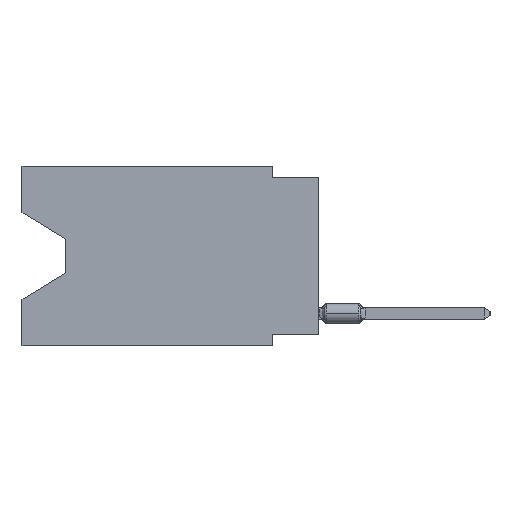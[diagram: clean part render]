
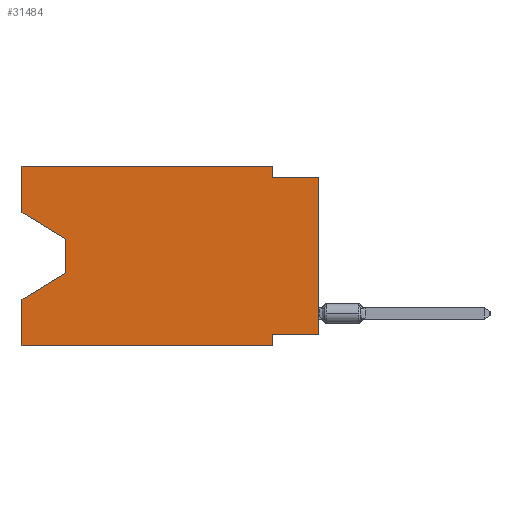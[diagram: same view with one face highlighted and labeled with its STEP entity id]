
A CAD part, left-side view. The second image highlights one B-rep face of the part: STEP entity #31484.
In plain terms, the highlighted planar face has unit normal (-1, 0, 0).
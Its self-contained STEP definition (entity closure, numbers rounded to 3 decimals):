
#155 = ORIENTED_EDGE ( 'NONE', *, *, #20727, .F. ) ;
#214 = AXIS2_PLACEMENT_3D ( 'NONE', #3123, #30117, #22687 ) ;
#402 = ORIENTED_EDGE ( 'NONE', *, *, #4136, .T. ) ;
#1003 = ORIENTED_EDGE ( 'NONE', *, *, #9504, .F. ) ;
#1324 = VECTOR ( 'NONE', #27673, 1000. ) ;
#1703 = LINE ( 'NONE', #6898, #7057 ) ;
#1825 = LINE ( 'NONE', #4101, #21482 ) ;
#2142 = DIRECTION ( 'NONE',  ( 0., 0., 1. ) ) ;
#2605 = CARTESIAN_POINT ( 'NONE',  ( 0., 16.383, 0. ) ) ;
#3123 = CARTESIAN_POINT ( 'NONE',  ( 0., 16.383, 0. ) ) ;
#3642 = VERTEX_POINT ( 'NONE', #16139 ) ;
#3894 = VECTOR ( 'NONE', #19125, 1000. ) ;
#3971 = DIRECTION ( 'NONE',  ( 0., -0.855, -0.519 ) ) ;
#4101 = CARTESIAN_POINT ( 'NONE',  ( 0., 16.383, 0. ) ) ;
#4132 = DIRECTION ( 'NONE',  ( 0., 0.855, -0.519 ) ) ;
#4136 = EDGE_CURVE ( 'NONE', #3642, #24219, #1703, .T. ) ;
#4231 = VERTEX_POINT ( 'NONE', #31960 ) ;
#4396 = LINE ( 'NONE', #24422, #4409 ) ;
#4409 = VECTOR ( 'NONE', #12322, 1000. ) ;
#5111 = EDGE_CURVE ( 'NONE', #23301, #28499, #31441, .T. ) ;
#5326 = VECTOR ( 'NONE', #3971, 1000. ) ;
#5373 = EDGE_CURVE ( 'NONE', #23481, #8202, #28333, .T. ) ;
#6181 = LINE ( 'NONE', #30898, #21129 ) ;
#6248 = CARTESIAN_POINT ( 'NONE',  ( 0., 2.54, -0.635 ) ) ;
#6339 = CARTESIAN_POINT ( 'NONE',  ( 0., 2.54, -9.271 ) ) ;
#6762 = CARTESIAN_POINT ( 'NONE',  ( 0., 0., -9.271 ) ) ;
#6898 = CARTESIAN_POINT ( 'NONE',  ( 0., 0., 0. ) ) ;
#7057 = VECTOR ( 'NONE', #25969, 1000. ) ;
#8122 = VERTEX_POINT ( 'NONE', #19099 ) ;
#8202 = VERTEX_POINT ( 'NONE', #22003 ) ;
#8298 = CARTESIAN_POINT ( 'NONE',  ( 0., 16.383, -7.36 ) ) ;
#8911 = VERTEX_POINT ( 'NONE', #6248 ) ;
#8922 = DIRECTION ( 'NONE',  ( 0., 0., -1. ) ) ;
#9165 = VERTEX_POINT ( 'NONE', #8298 ) ;
#9504 = EDGE_CURVE ( 'NONE', #13565, #8122, #4396, .T. ) ;
#11498 = ORIENTED_EDGE ( 'NONE', *, *, #24929, .F. ) ;
#12017 = ORIENTED_EDGE ( 'NONE', *, *, #30044, .T. ) ;
#12322 = DIRECTION ( 'NONE',  ( 0., 0., -1. ) ) ;
#13070 = EDGE_CURVE ( 'NONE', #18682, #9165, #1825, .T. ) ;
#13159 = FACE_OUTER_BOUND ( 'NONE', #25685, .T. ) ;
#13292 = ORIENTED_EDGE ( 'NONE', *, *, #21827, .F. ) ;
#13565 = VERTEX_POINT ( 'NONE', #6339 ) ;
#15362 = VECTOR ( 'NONE', #17952, 1000. ) ;
#16139 = CARTESIAN_POINT ( 'NONE',  ( 0., 0., -9.271 ) ) ;
#16423 = LINE ( 'NONE', #26285, #22925 ) ;
#16600 = DIRECTION ( 'NONE',  ( 0., 1., 0. ) ) ;
#16968 = CARTESIAN_POINT ( 'NONE',  ( 0., 0., -0.635 ) ) ;
#17156 = ORIENTED_EDGE ( 'NONE', *, *, #5111, .F. ) ;
#17716 = EDGE_CURVE ( 'NONE', #8202, #9165, #16423, .T. ) ;
#17952 = DIRECTION ( 'NONE',  ( 0., 0., 1. ) ) ;
#18466 = CARTESIAN_POINT ( 'NONE',  ( 0., 2.54, 0. ) ) ;
#18671 = LINE ( 'NONE', #21733, #5326 ) ;
#18682 = VERTEX_POINT ( 'NONE', #24848 ) ;
#19099 = CARTESIAN_POINT ( 'NONE',  ( 0., 2.54, -9.906 ) ) ;
#19125 = DIRECTION ( 'NONE',  ( 0., -1., 0. ) ) ;
#19732 = LINE ( 'NONE', #2605, #15362 ) ;
#19934 = CARTESIAN_POINT ( 'NONE',  ( 0., 13.97, -4.013 ) ) ;
#20142 = ORIENTED_EDGE ( 'NONE', *, *, #13070, .F. ) ;
#20372 = ORIENTED_EDGE ( 'NONE', *, *, #25924, .F. ) ;
#20727 = EDGE_CURVE ( 'NONE', #28499, #8911, #25898, .T. ) ;
#20994 = VECTOR ( 'NONE', #16600, 1000. ) ;
#21101 = CARTESIAN_POINT ( 'NONE',  ( 0., 16.383, 0. ) ) ;
#21112 = VECTOR ( 'NONE', #30807, 1000. ) ;
#21129 = VECTOR ( 'NONE', #23132, 1000. ) ;
#21482 = VECTOR ( 'NONE', #2142, 1000. ) ;
#21710 = CARTESIAN_POINT ( 'NONE',  ( 0., 16.383, 0. ) ) ;
#21733 = CARTESIAN_POINT ( 'NONE',  ( 0., 16.383, -2.546 ) ) ;
#21780 = ORIENTED_EDGE ( 'NONE', *, *, #17716, .T. ) ;
#21827 = EDGE_CURVE ( 'NONE', #8911, #24219, #25457, .T. ) ;
#22003 = CARTESIAN_POINT ( 'NONE',  ( 0., 13.97, -5.893 ) ) ;
#22291 = EDGE_CURVE ( 'NONE', #18682, #8122, #6181, .T. ) ;
#22601 = VECTOR ( 'NONE', #8922, 1000. ) ;
#22687 = DIRECTION ( 'NONE',  ( 0., 0., -1. ) ) ;
#22925 = VECTOR ( 'NONE', #4132, 1000. ) ;
#23132 = DIRECTION ( 'NONE',  ( 0., -1., 0. ) ) ;
#23301 = VERTEX_POINT ( 'NONE', #21101 ) ;
#23303 = CARTESIAN_POINT ( 'NONE',  ( 0., 13.97, -4.013 ) ) ;
#23481 = VERTEX_POINT ( 'NONE', #19934 ) ;
#24219 = VERTEX_POINT ( 'NONE', #16968 ) ;
#24422 = CARTESIAN_POINT ( 'NONE',  ( 0., 2.54, -9.906 ) ) ;
#24848 = CARTESIAN_POINT ( 'NONE',  ( 0., 16.383, -9.906 ) ) ;
#24929 = EDGE_CURVE ( 'NONE', #3642, #13565, #31642, .T. ) ;
#25119 = PLANE ( 'NONE',  #214 ) ;
#25457 = LINE ( 'NONE', #25797, #21112 ) ;
#25685 = EDGE_LOOP ( 'NONE', ( #12017, #29441, #21780, #20142, #28148, #1003, #11498, #402, #13292, #155, #17156, #20372 ) ) ;
#25797 = CARTESIAN_POINT ( 'NONE',  ( 0., 0., -0.635 ) ) ;
#25898 = LINE ( 'NONE', #18466, #22601 ) ;
#25924 = EDGE_CURVE ( 'NONE', #4231, #23301, #19732, .T. ) ;
#25969 = DIRECTION ( 'NONE',  ( 0., 0., 1. ) ) ;
#26285 = CARTESIAN_POINT ( 'NONE',  ( 0., 13.97, -5.893 ) ) ;
#27673 = DIRECTION ( 'NONE',  ( 0., 0., -1. ) ) ;
#28148 = ORIENTED_EDGE ( 'NONE', *, *, #22291, .T. ) ;
#28333 = LINE ( 'NONE', #23303, #1324 ) ;
#28499 = VERTEX_POINT ( 'NONE', #31499 ) ;
#29441 = ORIENTED_EDGE ( 'NONE', *, *, #5373, .T. ) ;
#30044 = EDGE_CURVE ( 'NONE', #4231, #23481, #18671, .T. ) ;
#30117 = DIRECTION ( 'NONE',  ( 1., 0., 0. ) ) ;
#30807 = DIRECTION ( 'NONE',  ( 0., -1., 0. ) ) ;
#30898 = CARTESIAN_POINT ( 'NONE',  ( 0., 16.383, -9.906 ) ) ;
#31441 = LINE ( 'NONE', #21710, #3894 ) ;
#31484 = ADVANCED_FACE ( 'NONE', ( #13159 ), #25119, .F. ) ;
#31499 = CARTESIAN_POINT ( 'NONE',  ( 0., 2.54, 0. ) ) ;
#31642 = LINE ( 'NONE', #6762, #20994 ) ;
#31960 = CARTESIAN_POINT ( 'NONE',  ( 0., 16.383, -2.546 ) ) ;
